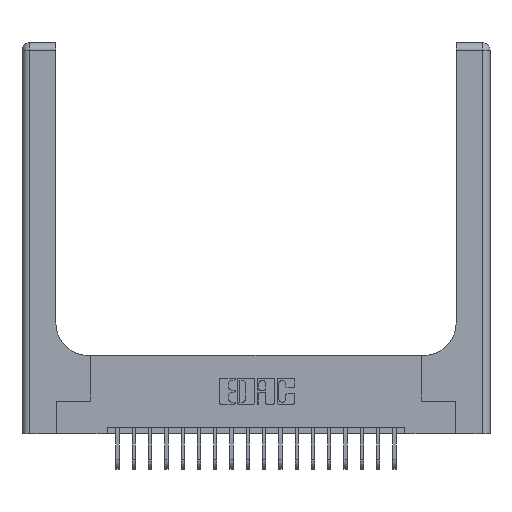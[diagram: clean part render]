
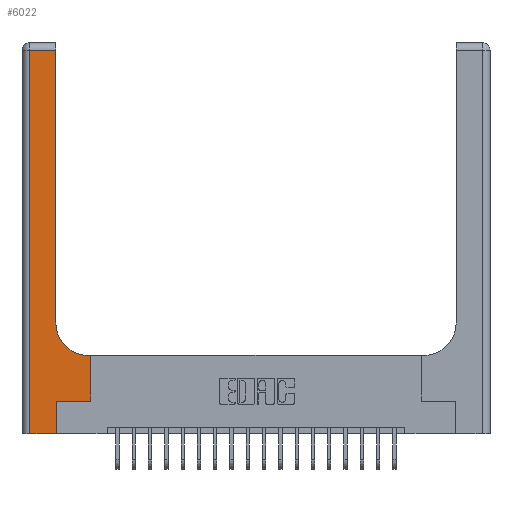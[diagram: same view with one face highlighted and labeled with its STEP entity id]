
A CAD part, top view. The second image highlights one B-rep face of the part: STEP entity #6022.
In plain terms, the highlighted planar face has unit normal (0, 0, 1).
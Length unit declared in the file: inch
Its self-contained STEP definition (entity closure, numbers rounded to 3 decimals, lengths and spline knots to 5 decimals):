
#594 = VERTEX_POINT ( 'NONE', #3985 ) ;
#878 = DIRECTION ( 'NONE',  ( 0., 0., -1. ) ) ;
#895 = ORIENTED_EDGE ( 'NONE', *, *, #19682, .T. ) ;
#995 = CARTESIAN_POINT ( 'NONE',  ( 0.265, 0.25, 0.37 ) ) ;
#1052 = EDGE_CURVE ( 'NONE', #16378, #1519, #4418, .T. ) ;
#1519 = VERTEX_POINT ( 'NONE', #11809 ) ;
#1761 = VERTEX_POINT ( 'NONE', #9424 ) ;
#1969 = DIRECTION ( 'NONE',  ( -1., 0., 0. ) ) ;
#2192 = ORIENTED_EDGE ( 'NONE', *, *, #18779, .T. ) ;
#2213 = CARTESIAN_POINT ( 'NONE',  ( 0.26, 0.6, 0.37 ) ) ;
#2278 = LINE ( 'NONE', #12536, #19510 ) ;
#3731 = CIRCLE ( 'NONE', #15818, 0.25 ) ;
#3832 = LINE ( 'NONE', #15869, #21314 ) ;
#3980 = VECTOR ( 'NONE', #14059, 39.37008 ) ;
#3985 = CARTESIAN_POINT ( 'NONE',  ( 0.26, 0.85, 0.37 ) ) ;
#4096 = DIRECTION ( 'NONE',  ( 0., -1., 0. ) ) ;
#4263 = LINE ( 'NONE', #21636, #21749 ) ;
#4418 = LINE ( 'NONE', #12624, #15290 ) ;
#4678 = DIRECTION ( 'NONE',  ( 1., 0., 0. ) ) ;
#5170 = ORIENTED_EDGE ( 'NONE', *, *, #8538, .T. ) ;
#5254 = VECTOR ( 'NONE', #11638, 39.37008 ) ;
#5422 = CARTESIAN_POINT ( 'NONE',  ( 0., 3., 0.37 ) ) ;
#5491 = PLANE ( 'NONE',  #8238 ) ;
#5648 = CARTESIAN_POINT ( 'NONE',  ( 0.528, 0.25, 0.37 ) ) ;
#5846 = DIRECTION ( 'NONE',  ( 1., 0., 0. ) ) ;
#5860 = DIRECTION ( 'NONE',  ( 0., 1., 0. ) ) ;
#6022 = ADVANCED_FACE ( 'NONE', ( #14867 ), #5491, .F. ) ;
#7651 = ORIENTED_EDGE ( 'NONE', *, *, #16948, .T. ) ;
#8097 = VERTEX_POINT ( 'NONE', #8487 ) ;
#8210 = VERTEX_POINT ( 'NONE', #17239 ) ;
#8238 = AXIS2_PLACEMENT_3D ( 'NONE', #5422, #12336, #1969 ) ;
#8314 = DIRECTION ( 'NONE',  ( 0., 1., 0. ) ) ;
#8487 = CARTESIAN_POINT ( 'NONE',  ( 0.265, 0., 0.37 ) ) ;
#8538 = EDGE_CURVE ( 'NONE', #8210, #8097, #2278, .T. ) ;
#9178 = CARTESIAN_POINT ( 'NONE',  ( 0.51, 0.85, 0.37 ) ) ;
#9424 = CARTESIAN_POINT ( 'NONE',  ( 0.51, 0.6, 0.37 ) ) ;
#9597 = VECTOR ( 'NONE', #20399, 39.37008 ) ;
#10151 = CARTESIAN_POINT ( 'NONE',  ( 0., 2.94, 0.37 ) ) ;
#10915 = CARTESIAN_POINT ( 'NONE',  ( 0.06, 2.94, 0.37 ) ) ;
#11479 = ORIENTED_EDGE ( 'NONE', *, *, #13166, .T. ) ;
#11638 = DIRECTION ( 'NONE',  ( -1., 0., 0. ) ) ;
#11655 = ORIENTED_EDGE ( 'NONE', *, *, #1052, .T. ) ;
#11809 = CARTESIAN_POINT ( 'NONE',  ( 0.528, 0.6, 0.37 ) ) ;
#11922 = EDGE_CURVE ( 'NONE', #8097, #16551, #17275, .T. ) ;
#12336 = DIRECTION ( 'NONE',  ( 0., 0., -1. ) ) ;
#12536 = CARTESIAN_POINT ( 'NONE',  ( 0., 0., 0.37 ) ) ;
#12624 = CARTESIAN_POINT ( 'NONE',  ( 0.528, 0.25, 0.37 ) ) ;
#12773 = VECTOR ( 'NONE', #8314, 39.37008 ) ;
#13025 = VERTEX_POINT ( 'NONE', #20513 ) ;
#13166 = EDGE_CURVE ( 'NONE', #1519, #1761, #16191, .T. ) ;
#13690 = EDGE_CURVE ( 'NONE', #1761, #594, #3731, .T. ) ;
#13869 = ORIENTED_EDGE ( 'NONE', *, *, #13690, .T. ) ;
#14059 = DIRECTION ( 'NONE',  ( -1., 0., 0. ) ) ;
#14867 = FACE_OUTER_BOUND ( 'NONE', #19568, .T. ) ;
#15003 = CARTESIAN_POINT ( 'NONE',  ( 0.265, 0., 0.37 ) ) ;
#15290 = VECTOR ( 'NONE', #5860, 39.37008 ) ;
#15818 = AXIS2_PLACEMENT_3D ( 'NONE', #9178, #878, #21106 ) ;
#15869 = CARTESIAN_POINT ( 'NONE',  ( 0.06, 3., 0.37 ) ) ;
#16191 = LINE ( 'NONE', #2213, #3980 ) ;
#16378 = VERTEX_POINT ( 'NONE', #5648 ) ;
#16551 = VERTEX_POINT ( 'NONE', #995 ) ;
#16948 = EDGE_CURVE ( 'NONE', #16961, #8210, #3832, .T. ) ;
#16961 = VERTEX_POINT ( 'NONE', #10915 ) ;
#16983 = CARTESIAN_POINT ( 'NONE',  ( 0.26, 3., 0.37 ) ) ;
#17239 = CARTESIAN_POINT ( 'NONE',  ( 0.06, 0., 0.37 ) ) ;
#17275 = LINE ( 'NONE', #15003, #12773 ) ;
#18779 = EDGE_CURVE ( 'NONE', #594, #13025, #19403, .T. ) ;
#19403 = LINE ( 'NONE', #16983, #9597 ) ;
#19510 = VECTOR ( 'NONE', #5846, 39.37008 ) ;
#19568 = EDGE_LOOP ( 'NONE', ( #2192, #20673, #7651, #5170, #20111, #895, #11655, #11479, #13869 ) ) ;
#19682 = EDGE_CURVE ( 'NONE', #16551, #16378, #4263, .T. ) ;
#20111 = ORIENTED_EDGE ( 'NONE', *, *, #11922, .T. ) ;
#20399 = DIRECTION ( 'NONE',  ( 0., 1., 0. ) ) ;
#20513 = CARTESIAN_POINT ( 'NONE',  ( 0.26, 2.94, 0.37 ) ) ;
#20673 = ORIENTED_EDGE ( 'NONE', *, *, #21628, .T. ) ;
#21106 = DIRECTION ( 'NONE',  ( 1., 0., 0. ) ) ;
#21157 = LINE ( 'NONE', #10151, #5254 ) ;
#21314 = VECTOR ( 'NONE', #4096, 39.37008 ) ;
#21628 = EDGE_CURVE ( 'NONE', #13025, #16961, #21157, .T. ) ;
#21636 = CARTESIAN_POINT ( 'NONE',  ( 0.265, 0.25, 0.37 ) ) ;
#21749 = VECTOR ( 'NONE', #4678, 39.37008 ) ;
